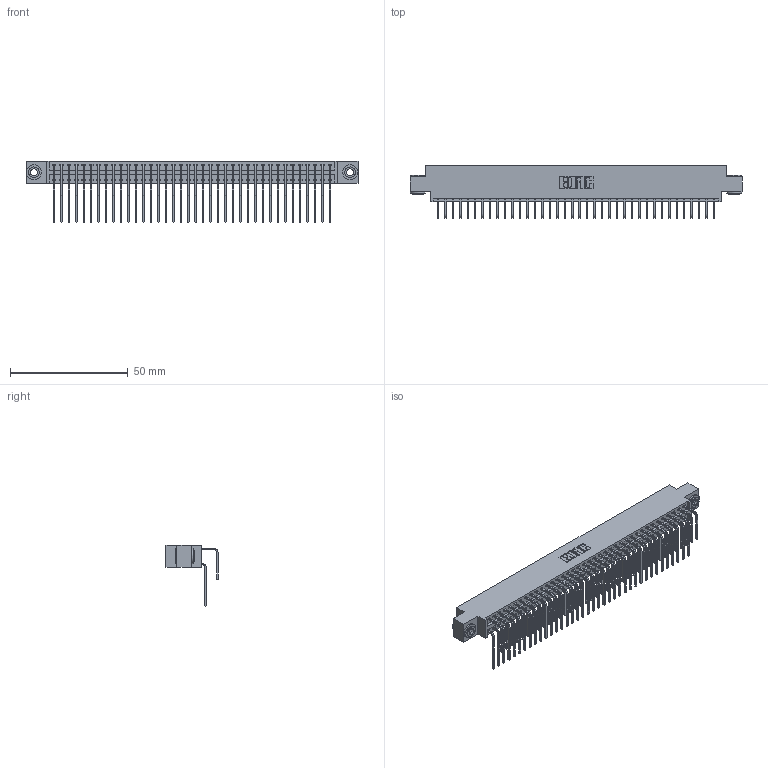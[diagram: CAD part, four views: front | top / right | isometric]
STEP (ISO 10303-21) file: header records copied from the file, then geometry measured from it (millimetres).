
FILE_DESCRIPTION (( 'STEP AP203' ), '1' );
FILE_NAME ('346-076-558-803.STEP', '2022-05-25T13:01:53', ( '' ), ( '' ), 'SwSTEP 2.0', 'SolidWorks 2020', '' );
FILE_SCHEMA (( 'CONFIG_CONTROL_DESIGN' ));
Length unit declared in the file: inch
Products named in the file (5): 346-076-558-803; 345-292-001_558 559 Tail - 1; 345-292-001_558 Tail - 2; 345-250-002_345-250-002-102; 346 Part_0.170 Offset - 0.156 Dia-TH
Assembly tree (79 placements, depth 2):
  346-076-558-803
    346 Part_0.170 Offset - 0.156 Dia-TH
    345-292-001_558 559 Tail - 1  x38
    345-292-001_558 Tail - 2  x38
    345-250-002_345-250-002-102  x2
Bounding box: 141.22 x 22.16 x 26.16 mm (x, y, z)
Volume: 14025.1 mm3; surface area: 21747.2 mm2
Topology: 79 solids, 79 shells, 4282 faces, 12689 edges, 8354 vertices
Faces by surface type: plane 2916, cylinder 1358, cone 8
Entity records: 28320 total; most frequent: CARTESIAN_POINT 4708, ORIENTED_EDGE 4582, DIRECTION 4201, EDGE_CURVE 2291, VECTOR 1943, LINE 1943, VERTEX_POINT 1522, AXIS2_PLACEMENT_3D 1129
